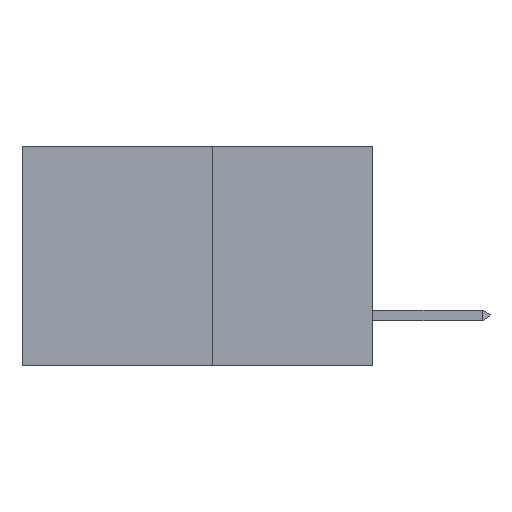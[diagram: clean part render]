
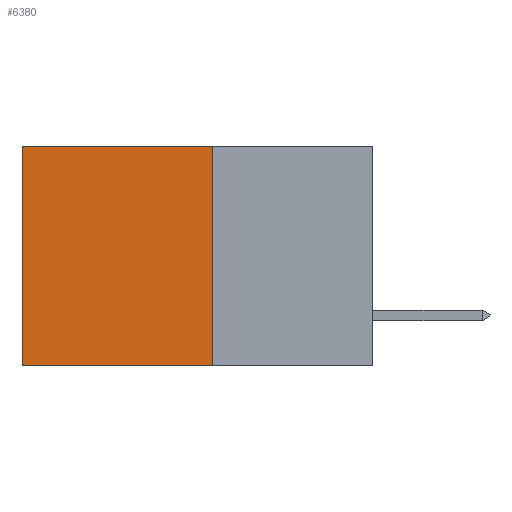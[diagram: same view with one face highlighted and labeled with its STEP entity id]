
A CAD part, left-side view. The second image highlights one B-rep face of the part: STEP entity #6380.
In plain terms, the highlighted planar face has unit normal (-1, 0, 0).
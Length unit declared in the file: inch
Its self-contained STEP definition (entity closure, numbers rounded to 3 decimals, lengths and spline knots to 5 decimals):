
#19 = AXIS2_PLACEMENT_3D ( 'NONE', #7721, #4974, #11153 ) ;
#138 = LINE ( 'NONE', #8664, #5140 ) ;
#564 = VERTEX_POINT ( 'NONE', #908 ) ;
#908 = CARTESIAN_POINT ( 'NONE',  ( 0.277, 0.59, 0. ) ) ;
#951 = DIRECTION ( 'NONE',  ( 0., 0., -1. ) ) ;
#1277 = LINE ( 'NONE', #7608, #3200 ) ;
#1892 = VECTOR ( 'NONE', #951, 39.37008 ) ;
#2164 = VECTOR ( 'NONE', #2250, 39.37008 ) ;
#2193 = LINE ( 'NONE', #10071, #1892 ) ;
#2250 = DIRECTION ( 'NONE',  ( 0., 1., 0. ) ) ;
#2739 = LINE ( 'NONE', #3174, #2164 ) ;
#3027 = DIRECTION ( 'NONE',  ( 0., 1., 0. ) ) ;
#3174 = CARTESIAN_POINT ( 'NONE',  ( 0.277, 0.27, -0.37 ) ) ;
#3200 = VECTOR ( 'NONE', #3027, 39.37008 ) ;
#3249 = DIRECTION ( 'NONE',  ( 0., 0., -1. ) ) ;
#4974 = DIRECTION ( 'NONE',  ( 1., 0., 0. ) ) ;
#5140 = VECTOR ( 'NONE', #3249, 39.37008 ) ;
#5705 = VERTEX_POINT ( 'NONE', #5983 ) ;
#5983 = CARTESIAN_POINT ( 'NONE',  ( 0.277, 0.27, -0.37 ) ) ;
#6015 = ORIENTED_EDGE ( 'NONE', *, *, #7956, .T. ) ;
#6289 = EDGE_CURVE ( 'NONE', #8518, #564, #1277, .T. ) ;
#6380 = ADVANCED_FACE ( 'NONE', ( #7234 ), #10307, .F. ) ;
#6433 = ORIENTED_EDGE ( 'NONE', *, *, #7689, .F. ) ;
#6786 = VERTEX_POINT ( 'NONE', #9200 ) ;
#7030 = EDGE_LOOP ( 'NONE', ( #6015, #9326, #6433, #7188 ) ) ;
#7036 = EDGE_CURVE ( 'NONE', #5705, #6786, #2739, .T. ) ;
#7188 = ORIENTED_EDGE ( 'NONE', *, *, #6289, .T. ) ;
#7234 = FACE_OUTER_BOUND ( 'NONE', #7030, .T. ) ;
#7608 = CARTESIAN_POINT ( 'NONE',  ( 0.277, 0.27, 0. ) ) ;
#7689 = EDGE_CURVE ( 'NONE', #8518, #5705, #138, .T. ) ;
#7721 = CARTESIAN_POINT ( 'NONE',  ( 0.277, 0.27, -0.37 ) ) ;
#7956 = EDGE_CURVE ( 'NONE', #564, #6786, #2193, .T. ) ;
#8518 = VERTEX_POINT ( 'NONE', #10827 ) ;
#8664 = CARTESIAN_POINT ( 'NONE',  ( 0.277, 0.27, -0.37 ) ) ;
#9200 = CARTESIAN_POINT ( 'NONE',  ( 0.277, 0.59, -0.37 ) ) ;
#9326 = ORIENTED_EDGE ( 'NONE', *, *, #7036, .F. ) ;
#10071 = CARTESIAN_POINT ( 'NONE',  ( 0.277, 0.59, -0.37 ) ) ;
#10307 = PLANE ( 'NONE',  #19 ) ;
#10827 = CARTESIAN_POINT ( 'NONE',  ( 0.277, 0.27, 0. ) ) ;
#11153 = DIRECTION ( 'NONE',  ( 0., 0., -1. ) ) ;
